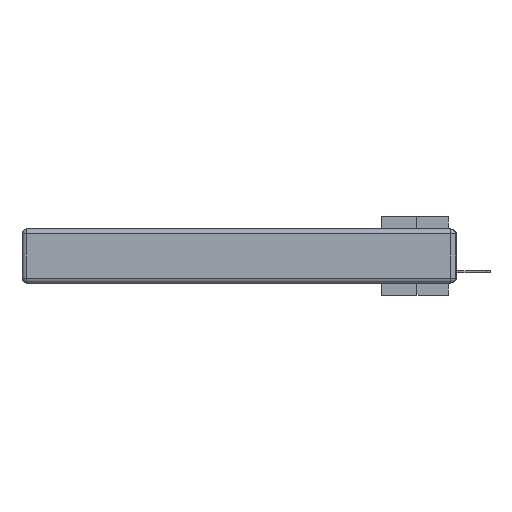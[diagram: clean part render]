
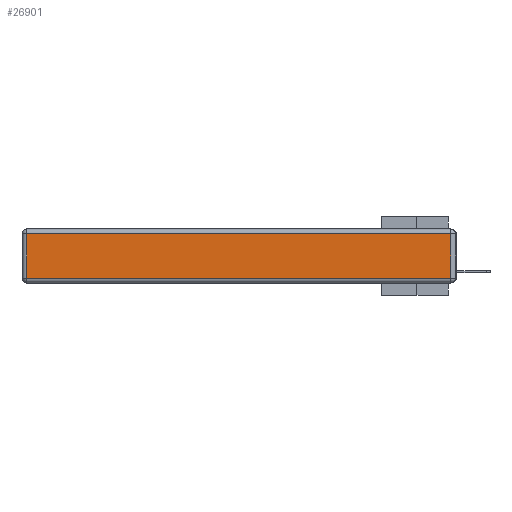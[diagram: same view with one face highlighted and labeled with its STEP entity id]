
A CAD part, left-side view. The second image highlights one B-rep face of the part: STEP entity #26901.
In plain terms, the highlighted planar face has unit normal (-1, 0, 0).
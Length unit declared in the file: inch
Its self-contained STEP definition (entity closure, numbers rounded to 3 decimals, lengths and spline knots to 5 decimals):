
#516 = AXIS2_PLACEMENT_3D ( 'NONE', #28571, #14835, #12476 ) ;
#816 = EDGE_CURVE ( 'NONE', #1862, #1905, #15278, .T. ) ;
#1862 = VERTEX_POINT ( 'NONE', #8341 ) ;
#1905 = VERTEX_POINT ( 'NONE', #12782 ) ;
#3726 = PLANE ( 'NONE',  #516 ) ;
#3938 = DIRECTION ( 'NONE',  ( 0., 0., 1. ) ) ;
#4771 = DIRECTION ( 'NONE',  ( 0., -1., 0. ) ) ;
#5996 = ORIENTED_EDGE ( 'NONE', *, *, #14315, .T. ) ;
#8170 = VERTEX_POINT ( 'NONE', #12913 ) ;
#8341 = CARTESIAN_POINT ( 'NONE',  ( 0., 2.72, -0.03 ) ) ;
#8460 = FACE_OUTER_BOUND ( 'NONE', #20554, .T. ) ;
#8914 = CARTESIAN_POINT ( 'NONE',  ( 0., 0., -0.313 ) ) ;
#8924 = CARTESIAN_POINT ( 'NONE',  ( 0., 2.72, -0.343 ) ) ;
#9217 = LINE ( 'NONE', #8914, #12247 ) ;
#11328 = EDGE_CURVE ( 'NONE', #8170, #17229, #26408, .T. ) ;
#12247 = VECTOR ( 'NONE', #4771, 39.37008 ) ;
#12476 = DIRECTION ( 'NONE',  ( 0., 0., 1. ) ) ;
#12687 = DIRECTION ( 'NONE',  ( 0., 1., 0. ) ) ;
#12782 = CARTESIAN_POINT ( 'NONE',  ( 0., 2.72, -0.313 ) ) ;
#12913 = CARTESIAN_POINT ( 'NONE',  ( 0., 0.03, -0.313 ) ) ;
#13801 = VECTOR ( 'NONE', #3938, 39.37008 ) ;
#14315 = EDGE_CURVE ( 'NONE', #17229, #1862, #17122, .T. ) ;
#14835 = DIRECTION ( 'NONE',  ( -1., 0., 0. ) ) ;
#15177 = CARTESIAN_POINT ( 'NONE',  ( 0., 0.03, -0.343 ) ) ;
#15278 = LINE ( 'NONE', #8924, #19415 ) ;
#16459 = ORIENTED_EDGE ( 'NONE', *, *, #816, .T. ) ;
#17122 = LINE ( 'NONE', #26149, #23328 ) ;
#17229 = VERTEX_POINT ( 'NONE', #17678 ) ;
#17678 = CARTESIAN_POINT ( 'NONE',  ( 0., 0.03, -0.03 ) ) ;
#19415 = VECTOR ( 'NONE', #26958, 39.37008 ) ;
#20554 = EDGE_LOOP ( 'NONE', ( #26931, #26129, #5996, #16459 ) ) ;
#21330 = EDGE_CURVE ( 'NONE', #1905, #8170, #9217, .T. ) ;
#23328 = VECTOR ( 'NONE', #12687, 39.37008 ) ;
#26129 = ORIENTED_EDGE ( 'NONE', *, *, #11328, .T. ) ;
#26149 = CARTESIAN_POINT ( 'NONE',  ( 0., 2.75, -0.03 ) ) ;
#26408 = LINE ( 'NONE', #15177, #13801 ) ;
#26901 = ADVANCED_FACE ( 'NONE', ( #8460 ), #3726, .T. ) ;
#26931 = ORIENTED_EDGE ( 'NONE', *, *, #21330, .T. ) ;
#26958 = DIRECTION ( 'NONE',  ( 0., 0., -1. ) ) ;
#28571 = CARTESIAN_POINT ( 'NONE',  ( 0., 0., -0.343 ) ) ;
